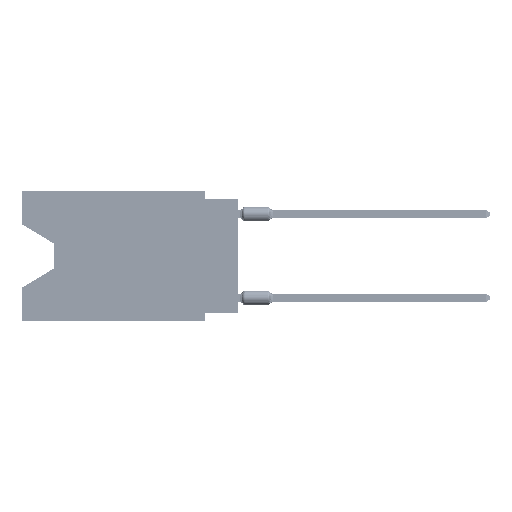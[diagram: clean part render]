
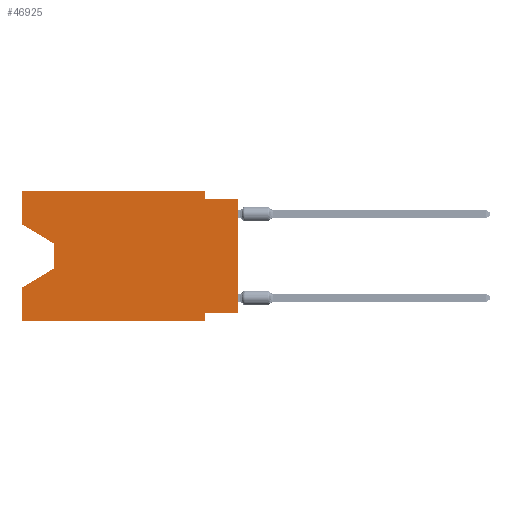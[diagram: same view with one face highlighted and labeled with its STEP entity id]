
A CAD part, left-side view. The second image highlights one B-rep face of the part: STEP entity #46925.
In plain terms, the highlighted planar face has unit normal (-1, 0, 0).
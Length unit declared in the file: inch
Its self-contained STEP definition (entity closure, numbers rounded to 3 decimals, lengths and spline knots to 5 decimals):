
#151 = ORIENTED_EDGE ( 'NONE', *, *, #47650, .F. ) ;
#295 = FACE_OUTER_BOUND ( 'NONE', #37935, .T. ) ;
#1593 = CARTESIAN_POINT ( 'NONE',  ( 0., 0.1, -0.365 ) ) ;
#3725 = CARTESIAN_POINT ( 'NONE',  ( 0., 0.1, 0. ) ) ;
#4037 = CARTESIAN_POINT ( 'NONE',  ( 0., 0., -0.365 ) ) ;
#4517 = EDGE_CURVE ( 'NONE', #34102, #22572, #73652, .T. ) ;
#8247 = CARTESIAN_POINT ( 'NONE',  ( 0., 0.645, -0.28975 ) ) ;
#8555 = VECTOR ( 'NONE', #46133, 39.37008 ) ;
#8738 = ORIENTED_EDGE ( 'NONE', *, *, #80007, .F. ) ;
#9288 = EDGE_CURVE ( 'NONE', #19491, #23977, #60795, .T. ) ;
#9759 = CARTESIAN_POINT ( 'NONE',  ( 0., 0.55, -0.158 ) ) ;
#9783 = DIRECTION ( 'NONE',  ( 0., -1., 0. ) ) ;
#11997 = EDGE_CURVE ( 'NONE', #65640, #23977, #26782, .T. ) ;
#13733 = ORIENTED_EDGE ( 'NONE', *, *, #54868, .T. ) ;
#14467 = CARTESIAN_POINT ( 'NONE',  ( 0., 0.1, -0.39 ) ) ;
#16081 = LINE ( 'NONE', #67332, #19954 ) ;
#16088 = DIRECTION ( 'NONE',  ( 0., -1., 0. ) ) ;
#16561 = LINE ( 'NONE', #53574, #22049 ) ;
#16854 = VERTEX_POINT ( 'NONE', #1593 ) ;
#17117 = CARTESIAN_POINT ( 'NONE',  ( 0., 0.1, -0.025 ) ) ;
#17523 = DIRECTION ( 'NONE',  ( 0., 0., 1. ) ) ;
#18082 = LINE ( 'NONE', #55485, #29404 ) ;
#18311 = CARTESIAN_POINT ( 'NONE',  ( 0., 0.1, 0. ) ) ;
#19491 = VERTEX_POINT ( 'NONE', #52799 ) ;
#19856 = CARTESIAN_POINT ( 'NONE',  ( 0., 0.55, -0.158 ) ) ;
#19954 = VECTOR ( 'NONE', #9783, 39.37008 ) ;
#22049 = VECTOR ( 'NONE', #34635, 39.37008 ) ;
#22572 = VERTEX_POINT ( 'NONE', #18311 ) ;
#23240 = VERTEX_POINT ( 'NONE', #19856 ) ;
#23243 = VECTOR ( 'NONE', #16088, 39.37008 ) ;
#23374 = CARTESIAN_POINT ( 'NONE',  ( 0., 0., 0. ) ) ;
#23977 = VERTEX_POINT ( 'NONE', #8247 ) ;
#25590 = VERTEX_POINT ( 'NONE', #14467 ) ;
#25933 = DIRECTION ( 'NONE',  ( 0., 0., -1. ) ) ;
#25935 = VECTOR ( 'NONE', #48584, 39.37008 ) ;
#25973 = VECTOR ( 'NONE', #42287, 39.37008 ) ;
#26782 = LINE ( 'NONE', #46116, #53623 ) ;
#27290 = CARTESIAN_POINT ( 'NONE',  ( 0., 0., -0.365 ) ) ;
#27336 = AXIS2_PLACEMENT_3D ( 'NONE', #46511, #38934, #25933 ) ;
#28816 = CARTESIAN_POINT ( 'NONE',  ( 0., 0., -0.025 ) ) ;
#29404 = VECTOR ( 'NONE', #37387, 39.37008 ) ;
#29555 = ORIENTED_EDGE ( 'NONE', *, *, #4517, .F. ) ;
#29734 = VERTEX_POINT ( 'NONE', #28816 ) ;
#29944 = VERTEX_POINT ( 'NONE', #82179 ) ;
#30090 = CARTESIAN_POINT ( 'NONE',  ( 0., 0.55, -0.232 ) ) ;
#30731 = LINE ( 'NONE', #9759, #68443 ) ;
#30962 = ORIENTED_EDGE ( 'NONE', *, *, #64038, .F. ) ;
#34102 = VERTEX_POINT ( 'NONE', #57458 ) ;
#34635 = DIRECTION ( 'NONE',  ( 0., 0., -1. ) ) ;
#34896 = ORIENTED_EDGE ( 'NONE', *, *, #49566, .F. ) ;
#37387 = DIRECTION ( 'NONE',  ( 0., -1., 0. ) ) ;
#37879 = EDGE_CURVE ( 'NONE', #23240, #19491, #30731, .T. ) ;
#37935 = EDGE_LOOP ( 'NONE', ( #72331, #75693, #50568, #39691, #13733, #151, #8738, #69446, #67163, #30962, #29555, #34896 ) ) ;
#38274 = CARTESIAN_POINT ( 'NONE',  ( 0., 0.645, 0. ) ) ;
#38934 = DIRECTION ( 'NONE',  ( 1., 0., 0. ) ) ;
#39691 = ORIENTED_EDGE ( 'NONE', *, *, #11997, .F. ) ;
#40796 = VERTEX_POINT ( 'NONE', #17117 ) ;
#42124 = CARTESIAN_POINT ( 'NONE',  ( 0., 0.645, 0. ) ) ;
#42287 = DIRECTION ( 'NONE',  ( 0., 0.855, -0.519 ) ) ;
#46116 = CARTESIAN_POINT ( 'NONE',  ( 0., 0.645, 0. ) ) ;
#46133 = DIRECTION ( 'NONE',  ( 0., -0.855, -0.519 ) ) ;
#46252 = DIRECTION ( 'NONE',  ( 0., 0., 1. ) ) ;
#46511 = CARTESIAN_POINT ( 'NONE',  ( 0., 0.645, 0. ) ) ;
#46925 = ADVANCED_FACE ( 'NONE', ( #295 ), #78030, .F. ) ;
#46961 = CARTESIAN_POINT ( 'NONE',  ( 0., 0.645, -0.10025 ) ) ;
#47033 = DIRECTION ( 'NONE',  ( 0., 1., 0. ) ) ;
#47650 = EDGE_CURVE ( 'NONE', #16854, #25590, #16561, .T. ) ;
#48584 = DIRECTION ( 'NONE',  ( 0., 0., 1. ) ) ;
#49566 = EDGE_CURVE ( 'NONE', #29944, #34102, #76532, .T. ) ;
#50339 = VECTOR ( 'NONE', #47033, 39.37008 ) ;
#50568 = ORIENTED_EDGE ( 'NONE', *, *, #9288, .T. ) ;
#52799 = CARTESIAN_POINT ( 'NONE',  ( 0., 0.55, -0.232 ) ) ;
#53351 = LINE ( 'NONE', #27290, #50339 ) ;
#53574 = CARTESIAN_POINT ( 'NONE',  ( 0., 0.1, -0.39 ) ) ;
#53623 = VECTOR ( 'NONE', #17523, 39.37008 ) ;
#54868 = EDGE_CURVE ( 'NONE', #65640, #25590, #16081, .T. ) ;
#55320 = LINE ( 'NONE', #23374, #25935 ) ;
#55485 = CARTESIAN_POINT ( 'NONE',  ( 0., 0., -0.025 ) ) ;
#57458 = CARTESIAN_POINT ( 'NONE',  ( 0., 0.645, 0. ) ) ;
#60795 = LINE ( 'NONE', #30090, #25973 ) ;
#61307 = LINE ( 'NONE', #3725, #64517 ) ;
#62563 = EDGE_CURVE ( 'NONE', #40796, #29734, #18082, .T. ) ;
#64038 = EDGE_CURVE ( 'NONE', #22572, #40796, #61307, .T. ) ;
#64517 = VECTOR ( 'NONE', #73898, 39.37008 ) ;
#65640 = VERTEX_POINT ( 'NONE', #74664 ) ;
#67163 = ORIENTED_EDGE ( 'NONE', *, *, #62563, .F. ) ;
#67332 = CARTESIAN_POINT ( 'NONE',  ( 0., 0.645, -0.39 ) ) ;
#67429 = VERTEX_POINT ( 'NONE', #4037 ) ;
#68151 = DIRECTION ( 'NONE',  ( 0., 0., -1. ) ) ;
#68443 = VECTOR ( 'NONE', #68151, 39.37008 ) ;
#68598 = EDGE_CURVE ( 'NONE', #29944, #23240, #72175, .T. ) ;
#69205 = VECTOR ( 'NONE', #46252, 39.37008 ) ;
#69446 = ORIENTED_EDGE ( 'NONE', *, *, #77960, .T. ) ;
#72175 = LINE ( 'NONE', #46961, #8555 ) ;
#72331 = ORIENTED_EDGE ( 'NONE', *, *, #68598, .T. ) ;
#73652 = LINE ( 'NONE', #42124, #23243 ) ;
#73898 = DIRECTION ( 'NONE',  ( 0., 0., -1. ) ) ;
#74664 = CARTESIAN_POINT ( 'NONE',  ( 0., 0.645, -0.39 ) ) ;
#75693 = ORIENTED_EDGE ( 'NONE', *, *, #37879, .T. ) ;
#76532 = LINE ( 'NONE', #38274, #69205 ) ;
#77960 = EDGE_CURVE ( 'NONE', #67429, #29734, #55320, .T. ) ;
#78030 = PLANE ( 'NONE',  #27336 ) ;
#80007 = EDGE_CURVE ( 'NONE', #67429, #16854, #53351, .T. ) ;
#82179 = CARTESIAN_POINT ( 'NONE',  ( 0., 0.645, -0.10025 ) ) ;
